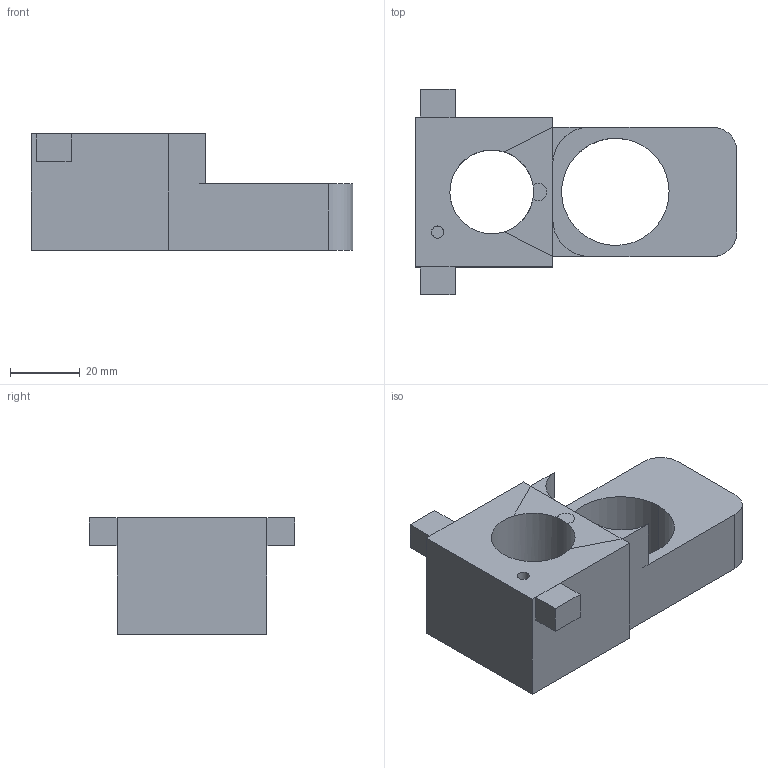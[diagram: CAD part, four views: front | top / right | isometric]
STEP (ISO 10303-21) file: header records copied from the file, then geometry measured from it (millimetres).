
FILE_DESCRIPTION(('FreeCAD Model'),'2;1');
FILE_NAME('buffer retainer.step', '2015-07-10T13:13:18',('Author'),(''), 'Open CASCADE STEP processor 6.8','FreeCAD','Unknown');
FILE_SCHEMA(('AUTOMOTIVE_DESIGN_CC2 { 1 2 10303 214 -1 1 5 4 }'));
Length unit declared in the file: millimetre
Products named in the file (1): Pocket008
Bounding box: 92.32 x 59 x 33.35 mm (x, y, z)
Volume: 65818 mm3; surface area: 18226.7 mm2
Topology: 1 solids, 1 shells, 49 faces, 122 edges, 79 vertices
Faces by surface type: plane 34, cylinder 15
Full cylindrical faces by diameter (mm): 2.5 x4, 3.5 x1, 24 x1
Entity records: 3102 total; most frequent: CARTESIAN_POINT 674, DIRECTION 441, ORIENTED_EDGE 244, PCURVE 244, DEFINITIONAL_REPRESENTATION 244, LINE 244, VECTOR 244, EDGE_CURVE 122
